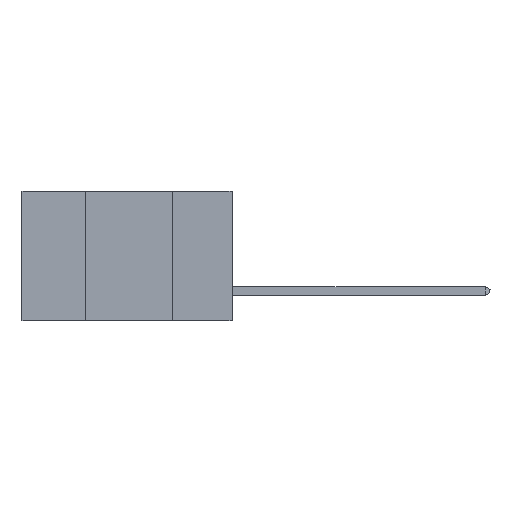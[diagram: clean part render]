
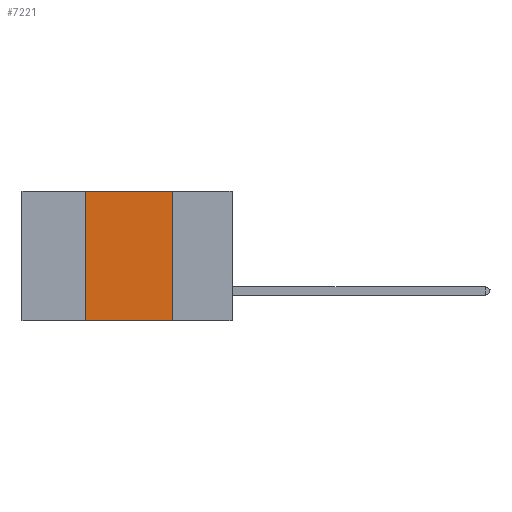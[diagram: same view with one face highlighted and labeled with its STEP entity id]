
A CAD part, left-side view. The second image highlights one B-rep face of the part: STEP entity #7221.
In plain terms, the highlighted planar face has unit normal (-1, 0, 0).
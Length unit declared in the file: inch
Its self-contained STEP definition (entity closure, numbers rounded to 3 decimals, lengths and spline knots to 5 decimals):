
#44 = CARTESIAN_POINT ( 'NONE',  ( 0., 0.42, 0. ) ) ;
#1698 = EDGE_CURVE ( 'NONE', #12024, #37046, #37438, .T. ) ;
#2466 = CARTESIAN_POINT ( 'NONE',  ( 0., 0.17, 0. ) ) ;
#3060 = AXIS2_PLACEMENT_3D ( 'NONE', #12905, #36909, #34130 ) ;
#4071 = EDGE_CURVE ( 'NONE', #12611, #12024, #29734, .T. ) ;
#4152 = ORIENTED_EDGE ( 'NONE', *, *, #34134, .F. ) ;
#4471 = DIRECTION ( 'NONE',  ( 0., 0., -1. ) ) ;
#5457 = DIRECTION ( 'NONE',  ( 0., 0., 1. ) ) ;
#5713 = LINE ( 'NONE', #8399, #36223 ) ;
#7221 = ADVANCED_FACE ( 'NONE', ( #15653 ), #30837, .F. ) ;
#8399 = CARTESIAN_POINT ( 'NONE',  ( 0., 0.6, -0.37 ) ) ;
#9440 = EDGE_LOOP ( 'NONE', ( #4152, #12062, #36089, #20970 ) ) ;
#12024 = VERTEX_POINT ( 'NONE', #44 ) ;
#12062 = ORIENTED_EDGE ( 'NONE', *, *, #1698, .F. ) ;
#12611 = VERTEX_POINT ( 'NONE', #29792 ) ;
#12905 = CARTESIAN_POINT ( 'NONE',  ( 0., 0.6, 0. ) ) ;
#13816 = CARTESIAN_POINT ( 'NONE',  ( 0., 0.17, 0. ) ) ;
#14161 = CARTESIAN_POINT ( 'NONE',  ( 0., 0.6, 0. ) ) ;
#14728 = EDGE_CURVE ( 'NONE', #12611, #21329, #5713, .T. ) ;
#15653 = FACE_OUTER_BOUND ( 'NONE', #9440, .T. ) ;
#20970 = ORIENTED_EDGE ( 'NONE', *, *, #14728, .T. ) ;
#21329 = VERTEX_POINT ( 'NONE', #34797 ) ;
#23407 = CARTESIAN_POINT ( 'NONE',  ( 0., 0.42, 0. ) ) ;
#29344 = DIRECTION ( 'NONE',  ( 0., -1., 0. ) ) ;
#29734 = LINE ( 'NONE', #23407, #35862 ) ;
#29792 = CARTESIAN_POINT ( 'NONE',  ( 0., 0.42, -0.37 ) ) ;
#30411 = VECTOR ( 'NONE', #4471, 39.37008 ) ;
#30837 = PLANE ( 'NONE',  #3060 ) ;
#31870 = LINE ( 'NONE', #13816, #30411 ) ;
#34130 = DIRECTION ( 'NONE',  ( 0., 0., -1. ) ) ;
#34134 = EDGE_CURVE ( 'NONE', #37046, #21329, #31870, .T. ) ;
#34149 = VECTOR ( 'NONE', #35127, 39.37008 ) ;
#34797 = CARTESIAN_POINT ( 'NONE',  ( 0., 0.17, -0.37 ) ) ;
#35127 = DIRECTION ( 'NONE',  ( 0., -1., 0. ) ) ;
#35862 = VECTOR ( 'NONE', #5457, 39.37008 ) ;
#36089 = ORIENTED_EDGE ( 'NONE', *, *, #4071, .F. ) ;
#36223 = VECTOR ( 'NONE', #29344, 39.37008 ) ;
#36909 = DIRECTION ( 'NONE',  ( 1., 0., 0. ) ) ;
#37046 = VERTEX_POINT ( 'NONE', #2466 ) ;
#37438 = LINE ( 'NONE', #14161, #34149 ) ;
